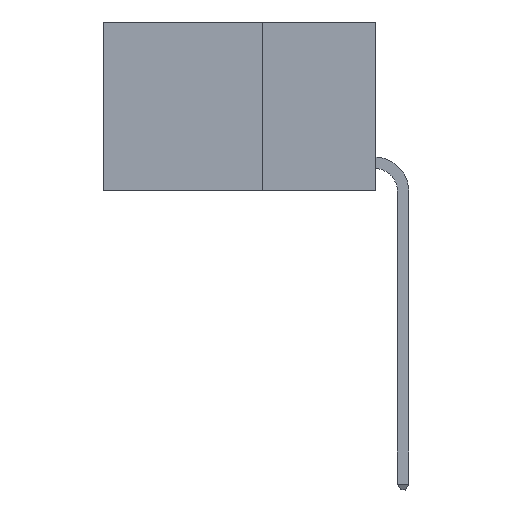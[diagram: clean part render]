
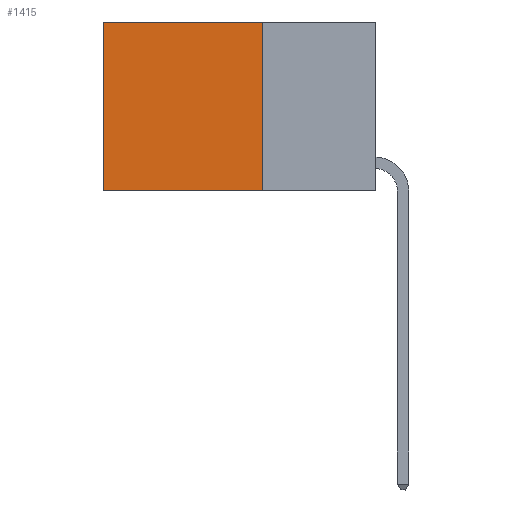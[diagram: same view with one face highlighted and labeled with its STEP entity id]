
A CAD part, left-side view. The second image highlights one B-rep face of the part: STEP entity #1415.
In plain terms, the highlighted planar face has unit normal (-1, 0, 0).
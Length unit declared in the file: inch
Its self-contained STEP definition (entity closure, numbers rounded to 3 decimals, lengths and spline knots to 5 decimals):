
#363 = CARTESIAN_POINT ( 'NONE',  ( 0.2625, 0.6, -0.37 ) ) ;
#439 = EDGE_LOOP ( 'NONE', ( #11949, #1023, #9457, #7102 ) ) ;
#1023 = ORIENTED_EDGE ( 'NONE', *, *, #10099, .F. ) ;
#1192 = CARTESIAN_POINT ( 'NONE',  ( 0.2625, 0.25, 0. ) ) ;
#1250 = CARTESIAN_POINT ( 'NONE',  ( 0.2625, 0.25, -0.37 ) ) ;
#1401 = VERTEX_POINT ( 'NONE', #5058 ) ;
#1415 = ADVANCED_FACE ( 'NONE', ( #3570 ), #8255, .F. ) ;
#2121 = LINE ( 'NONE', #1192, #4728 ) ;
#2182 = DIRECTION ( 'NONE',  ( 0., 1., 0. ) ) ;
#2356 = DIRECTION ( 'NONE',  ( 0., 0., -1. ) ) ;
#3570 = FACE_OUTER_BOUND ( 'NONE', #439, .T. ) ;
#4210 = EDGE_CURVE ( 'NONE', #1401, #6927, #2121, .T. ) ;
#4643 = VECTOR ( 'NONE', #10868, 39.37008 ) ;
#4728 = VECTOR ( 'NONE', #2356, 39.37008 ) ;
#5058 = CARTESIAN_POINT ( 'NONE',  ( 0.2625, 0.25, 0. ) ) ;
#5493 = AXIS2_PLACEMENT_3D ( 'NONE', #13184, #11205, #9249 ) ;
#6801 = CARTESIAN_POINT ( 'NONE',  ( 0.2625, 0.25, -0.37 ) ) ;
#6927 = VERTEX_POINT ( 'NONE', #1250 ) ;
#7014 = LINE ( 'NONE', #8508, #12629 ) ;
#7102 = ORIENTED_EDGE ( 'NONE', *, *, #10615, .T. ) ;
#7133 = VERTEX_POINT ( 'NONE', #11141 ) ;
#7188 = LINE ( 'NONE', #6801, #4643 ) ;
#8255 = PLANE ( 'NONE',  #5493 ) ;
#8508 = CARTESIAN_POINT ( 'NONE',  ( 0.2625, 0.6, 0. ) ) ;
#8617 = CARTESIAN_POINT ( 'NONE',  ( 0.2625, 0.25, 0. ) ) ;
#8904 = VECTOR ( 'NONE', #2182, 39.37008 ) ;
#8979 = VERTEX_POINT ( 'NONE', #363 ) ;
#9249 = DIRECTION ( 'NONE',  ( 0., 0., -1. ) ) ;
#9457 = ORIENTED_EDGE ( 'NONE', *, *, #4210, .F. ) ;
#9509 = DIRECTION ( 'NONE',  ( 0., 0., -1. ) ) ;
#9897 = EDGE_CURVE ( 'NONE', #7133, #8979, #7014, .T. ) ;
#10099 = EDGE_CURVE ( 'NONE', #6927, #8979, #7188, .T. ) ;
#10615 = EDGE_CURVE ( 'NONE', #1401, #7133, #11225, .T. ) ;
#10868 = DIRECTION ( 'NONE',  ( 0., 1., 0. ) ) ;
#11141 = CARTESIAN_POINT ( 'NONE',  ( 0.2625, 0.6, 0. ) ) ;
#11205 = DIRECTION ( 'NONE',  ( 1., 0., 0. ) ) ;
#11225 = LINE ( 'NONE', #8617, #8904 ) ;
#11949 = ORIENTED_EDGE ( 'NONE', *, *, #9897, .T. ) ;
#12629 = VECTOR ( 'NONE', #9509, 39.37008 ) ;
#13184 = CARTESIAN_POINT ( 'NONE',  ( 0.2625, 0.25, 0. ) ) ;
